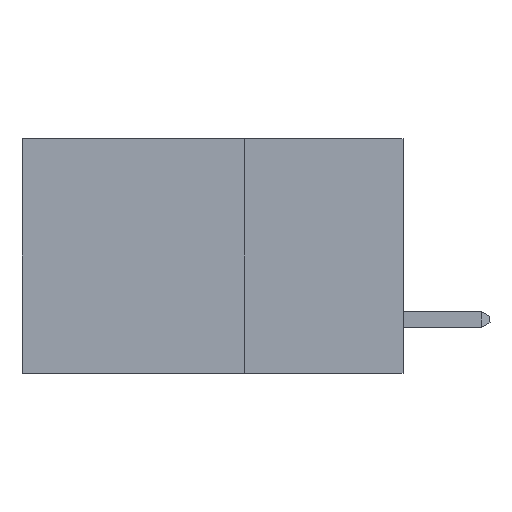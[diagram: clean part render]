
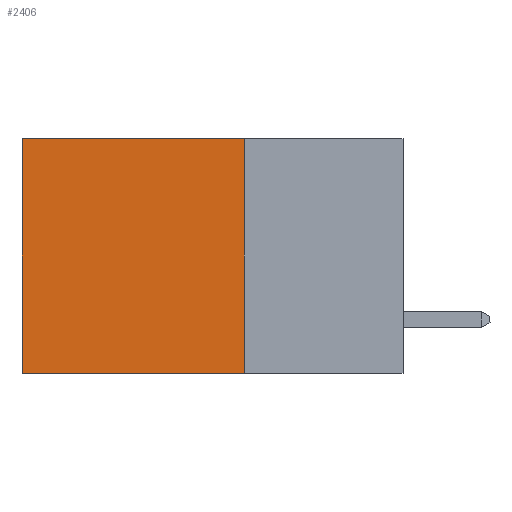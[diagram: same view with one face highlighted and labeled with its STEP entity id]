
A CAD part, left-side view. The second image highlights one B-rep face of the part: STEP entity #2406.
In plain terms, the highlighted planar face has unit normal (-1, 0, 0).
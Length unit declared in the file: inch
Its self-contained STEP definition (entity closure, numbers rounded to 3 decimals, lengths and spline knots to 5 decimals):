
#41 = LINE ( 'NONE', #4888, #9144 ) ;
#740 = DIRECTION ( 'NONE',  ( 1., 0., 0. ) ) ;
#2406 = ADVANCED_FACE ( 'NONE', ( #14630 ), #10089, .F. ) ;
#2441 = DIRECTION ( 'NONE',  ( 0., 1., 0. ) ) ;
#2760 = ORIENTED_EDGE ( 'NONE', *, *, #4172, .T. ) ;
#3123 = CARTESIAN_POINT ( 'NONE',  ( 0.2875, 0.25, -0.37 ) ) ;
#3445 = VECTOR ( 'NONE', #2441, 39.37008 ) ;
#3462 = EDGE_LOOP ( 'NONE', ( #2760, #12502, #10399, #6257 ) ) ;
#3503 = VERTEX_POINT ( 'NONE', #6527 ) ;
#3967 = LINE ( 'NONE', #12466, #12339 ) ;
#4172 = EDGE_CURVE ( 'NONE', #3503, #5557, #5733, .T. ) ;
#4853 = VERTEX_POINT ( 'NONE', #3123 ) ;
#4888 = CARTESIAN_POINT ( 'NONE',  ( 0.2875, 0.25, 0. ) ) ;
#5557 = VERTEX_POINT ( 'NONE', #10218 ) ;
#5719 = EDGE_CURVE ( 'NONE', #4853, #5557, #9945, .T. ) ;
#5733 = LINE ( 'NONE', #11845, #14279 ) ;
#6257 = ORIENTED_EDGE ( 'NONE', *, *, #6735, .T. ) ;
#6527 = CARTESIAN_POINT ( 'NONE',  ( 0.2875, 0.6, 0. ) ) ;
#6735 = EDGE_CURVE ( 'NONE', #11946, #3503, #3967, .T. ) ;
#8263 = CARTESIAN_POINT ( 'NONE',  ( 0.2875, 0.25, -0.37 ) ) ;
#8982 = DIRECTION ( 'NONE',  ( 0., 0., -1. ) ) ;
#9144 = VECTOR ( 'NONE', #9413, 39.37008 ) ;
#9413 = DIRECTION ( 'NONE',  ( 0., 0., -1. ) ) ;
#9945 = LINE ( 'NONE', #8263, #3445 ) ;
#10089 = PLANE ( 'NONE',  #11170 ) ;
#10218 = CARTESIAN_POINT ( 'NONE',  ( 0.2875, 0.6, -0.37 ) ) ;
#10399 = ORIENTED_EDGE ( 'NONE', *, *, #12472, .F. ) ;
#10735 = DIRECTION ( 'NONE',  ( 0., 0., -1. ) ) ;
#11170 = AXIS2_PLACEMENT_3D ( 'NONE', #13398, #740, #8982 ) ;
#11384 = DIRECTION ( 'NONE',  ( 0., 1., 0. ) ) ;
#11845 = CARTESIAN_POINT ( 'NONE',  ( 0.2875, 0.6, 0. ) ) ;
#11946 = VERTEX_POINT ( 'NONE', #13047 ) ;
#12339 = VECTOR ( 'NONE', #11384, 39.37008 ) ;
#12466 = CARTESIAN_POINT ( 'NONE',  ( 0.2875, 0.25, 0. ) ) ;
#12472 = EDGE_CURVE ( 'NONE', #11946, #4853, #41, .T. ) ;
#12502 = ORIENTED_EDGE ( 'NONE', *, *, #5719, .F. ) ;
#13047 = CARTESIAN_POINT ( 'NONE',  ( 0.2875, 0.25, 0. ) ) ;
#13398 = CARTESIAN_POINT ( 'NONE',  ( 0.2875, 0.25, 0. ) ) ;
#14279 = VECTOR ( 'NONE', #10735, 39.37008 ) ;
#14630 = FACE_OUTER_BOUND ( 'NONE', #3462, .T. ) ;
